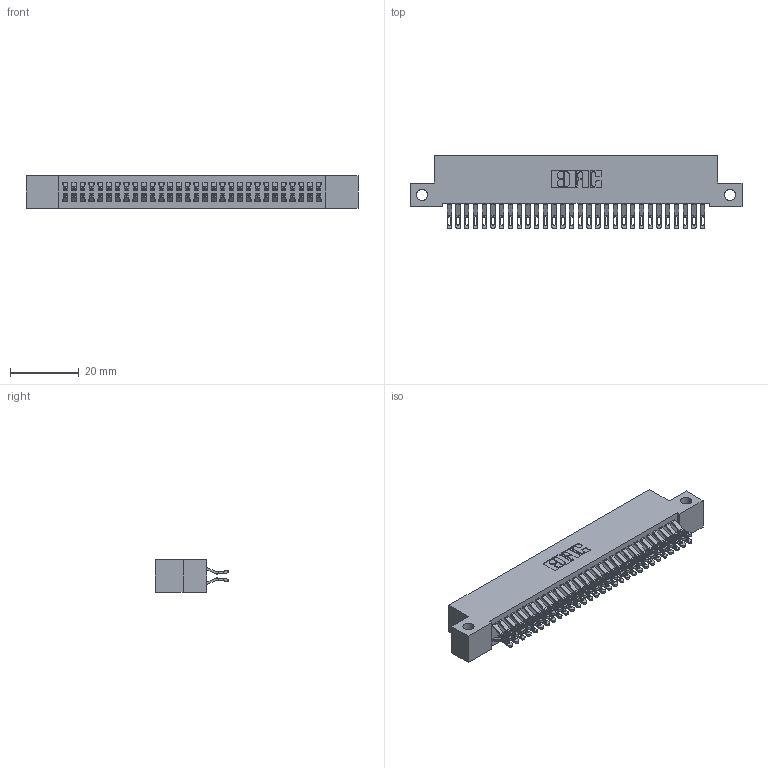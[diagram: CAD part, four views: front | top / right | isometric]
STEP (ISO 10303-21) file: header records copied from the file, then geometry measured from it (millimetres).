
FILE_DESCRIPTION (( 'STEP AP203' ), '1' );
FILE_NAME ('342-060-555-212.STEP', '2018-08-13T06:18:23', ( '' ), ( '' ), 'SwSTEP 2.0', 'SolidWorks 2016', '' );
FILE_SCHEMA (( 'CONFIG_CONTROL_DESIGN' ));
Length unit declared in the file: inch
Products named in the file (3): 342 Part_Side Mount; 345-292-001_555 Tail; 342-060-555-212
Assembly tree (61 placements, depth 2):
  342-060-555-212
    342 Part_Side Mount
    345-292-001_555 Tail  x60
Bounding box: 96.52 x 21.47 x 9.4 mm (x, y, z)
Volume: 8708.3 mm3; surface area: 14300 mm2
Topology: 61 solids, 61 shells, 3590 faces, 11279 edges, 7518 vertices
Faces by surface type: plane 2106, cylinder 1484
Entity records: 21049 total; most frequent: CARTESIAN_POINT 3536, ORIENTED_EDGE 3442, DIRECTION 3013, EDGE_CURVE 1721, VECTOR 1573, LINE 1573, VERTEX_POINT 1146, AXIS2_PLACEMENT_3D 720
